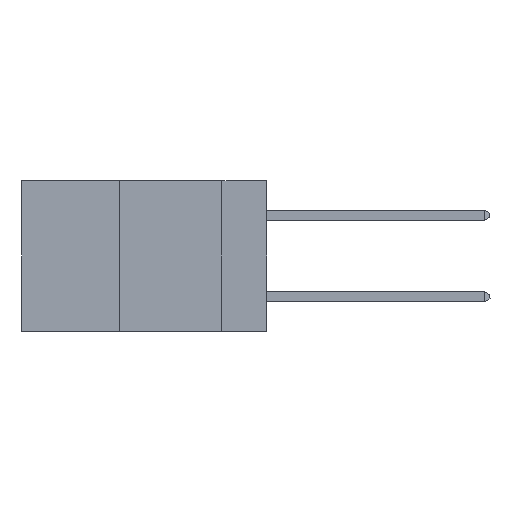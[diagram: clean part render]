
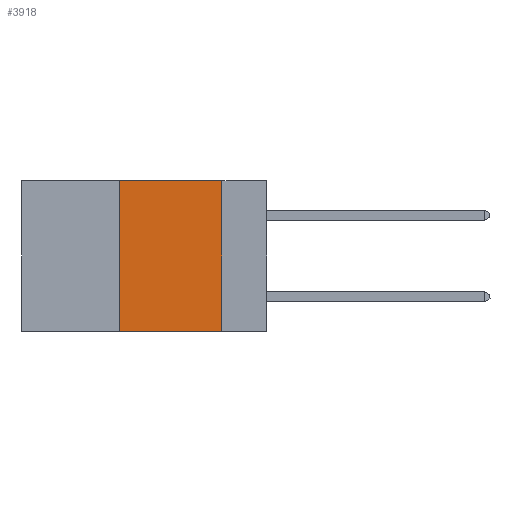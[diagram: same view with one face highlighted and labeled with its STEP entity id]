
A CAD part, left-side view. The second image highlights one B-rep face of the part: STEP entity #3918.
In plain terms, the highlighted planar face has unit normal (-1, 0, 0).
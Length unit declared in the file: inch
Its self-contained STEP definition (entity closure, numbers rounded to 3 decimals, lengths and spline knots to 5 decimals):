
#456 = CARTESIAN_POINT ( 'NONE',  ( 0., 0.6, -0.37 ) ) ;
#755 = DIRECTION ( 'NONE',  ( 0., 0., -1. ) ) ;
#1119 = ORIENTED_EDGE ( 'NONE', *, *, #4443, .F. ) ;
#2583 = EDGE_CURVE ( 'NONE', #16904, #11293, #10748, .T. ) ;
#2837 = LINE ( 'NONE', #7721, #17232 ) ;
#3918 = ADVANCED_FACE ( 'NONE', ( #15971 ), #6234, .F. ) ;
#3952 = VECTOR ( 'NONE', #13948, 39.37008 ) ;
#4443 = EDGE_CURVE ( 'NONE', #13160, #16904, #7248, .T. ) ;
#5187 = CARTESIAN_POINT ( 'NONE',  ( 0., 0.36, -0.37 ) ) ;
#6204 = EDGE_LOOP ( 'NONE', ( #17045, #6783, #1119, #12658 ) ) ;
#6234 = PLANE ( 'NONE',  #12947 ) ;
#6293 = CARTESIAN_POINT ( 'NONE',  ( 0., 0.6, 0. ) ) ;
#6783 = ORIENTED_EDGE ( 'NONE', *, *, #2583, .F. ) ;
#7060 = CARTESIAN_POINT ( 'NONE',  ( 0., 0.36, 0. ) ) ;
#7061 = VECTOR ( 'NONE', #17135, 39.37008 ) ;
#7248 = LINE ( 'NONE', #7060, #3952 ) ;
#7355 = DIRECTION ( 'NONE',  ( 0., -1., 0. ) ) ;
#7721 = CARTESIAN_POINT ( 'NONE',  ( 0., 0.11, 0. ) ) ;
#9100 = DIRECTION ( 'NONE',  ( 1., 0., 0. ) ) ;
#9108 = DIRECTION ( 'NONE',  ( 0., 0., -1. ) ) ;
#10473 = LINE ( 'NONE', #456, #17452 ) ;
#10748 = LINE ( 'NONE', #12899, #7061 ) ;
#10753 = CARTESIAN_POINT ( 'NONE',  ( 0., 0.36, 0. ) ) ;
#10944 = VERTEX_POINT ( 'NONE', #12745 ) ;
#11038 = EDGE_CURVE ( 'NONE', #13160, #10944, #10473, .T. ) ;
#11293 = VERTEX_POINT ( 'NONE', #16540 ) ;
#12658 = ORIENTED_EDGE ( 'NONE', *, *, #11038, .T. ) ;
#12745 = CARTESIAN_POINT ( 'NONE',  ( 0., 0.11, -0.37 ) ) ;
#12899 = CARTESIAN_POINT ( 'NONE',  ( 0., 0.6, 0. ) ) ;
#12947 = AXIS2_PLACEMENT_3D ( 'NONE', #6293, #9100, #755 ) ;
#13032 = EDGE_CURVE ( 'NONE', #11293, #10944, #2837, .T. ) ;
#13160 = VERTEX_POINT ( 'NONE', #5187 ) ;
#13948 = DIRECTION ( 'NONE',  ( 0., 0., 1. ) ) ;
#15971 = FACE_OUTER_BOUND ( 'NONE', #6204, .T. ) ;
#16540 = CARTESIAN_POINT ( 'NONE',  ( 0., 0.11, 0. ) ) ;
#16904 = VERTEX_POINT ( 'NONE', #10753 ) ;
#17045 = ORIENTED_EDGE ( 'NONE', *, *, #13032, .F. ) ;
#17135 = DIRECTION ( 'NONE',  ( 0., -1., 0. ) ) ;
#17232 = VECTOR ( 'NONE', #9108, 39.37008 ) ;
#17452 = VECTOR ( 'NONE', #7355, 39.37008 ) ;
